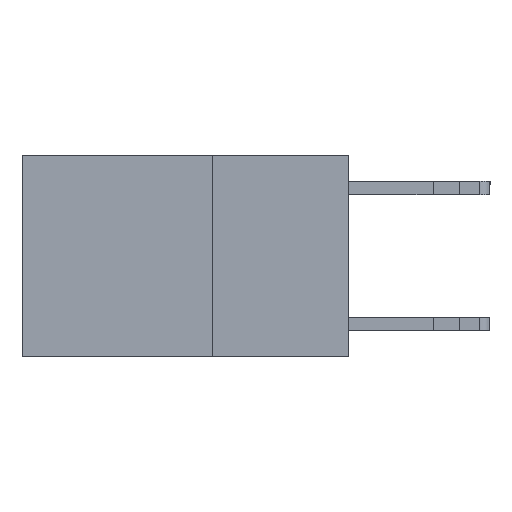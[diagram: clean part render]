
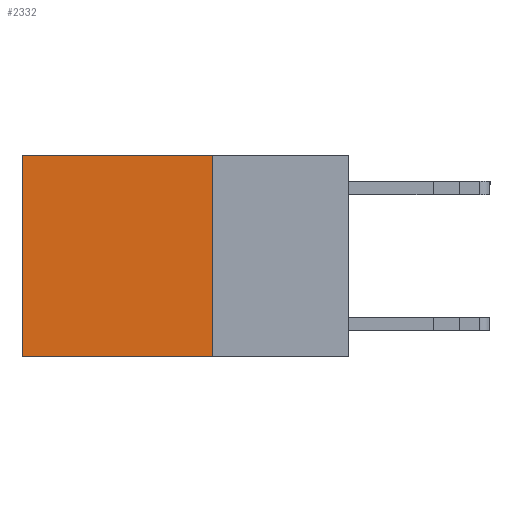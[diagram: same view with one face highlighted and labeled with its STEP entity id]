
A CAD part, left-side view. The second image highlights one B-rep face of the part: STEP entity #2332.
In plain terms, the highlighted planar face has unit normal (-1, 0, 0).
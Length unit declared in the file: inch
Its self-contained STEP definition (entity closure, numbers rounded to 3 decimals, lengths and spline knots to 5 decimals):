
#118 = ORIENTED_EDGE ( 'NONE', *, *, #10918, .F. ) ;
#354 = EDGE_LOOP ( 'NONE', ( #3992, #118, #1312, #5912 ) ) ;
#703 = CARTESIAN_POINT ( 'NONE',  ( 0.2625, 0.25, -0.37 ) ) ;
#1312 = ORIENTED_EDGE ( 'NONE', *, *, #5568, .F. ) ;
#1367 = DIRECTION ( 'NONE',  ( 1., 0., 0. ) ) ;
#1908 = DIRECTION ( 'NONE',  ( 0., 1., 0. ) ) ;
#2332 = ADVANCED_FACE ( 'NONE', ( #8041 ), #6846, .F. ) ;
#2643 = CARTESIAN_POINT ( 'NONE',  ( 0.2625, 0.25, 0. ) ) ;
#2870 = LINE ( 'NONE', #10393, #11684 ) ;
#3019 = EDGE_CURVE ( 'NONE', #7114, #11416, #11569, .T. ) ;
#3902 = AXIS2_PLACEMENT_3D ( 'NONE', #2643, #1367, #10035 ) ;
#3992 = ORIENTED_EDGE ( 'NONE', *, *, #6946, .T. ) ;
#4894 = DIRECTION ( 'NONE',  ( 0., 1., 0. ) ) ;
#5568 = EDGE_CURVE ( 'NONE', #7114, #9580, #7839, .T. ) ;
#5912 = ORIENTED_EDGE ( 'NONE', *, *, #3019, .T. ) ;
#6136 = DIRECTION ( 'NONE',  ( 0., 0., -1. ) ) ;
#6617 = VECTOR ( 'NONE', #11100, 39.37008 ) ;
#6784 = CARTESIAN_POINT ( 'NONE',  ( 0.2625, 0.25, 0. ) ) ;
#6846 = PLANE ( 'NONE',  #3902 ) ;
#6946 = EDGE_CURVE ( 'NONE', #11416, #12065, #2870, .T. ) ;
#7114 = VERTEX_POINT ( 'NONE', #9755 ) ;
#7839 = LINE ( 'NONE', #6784, #6617 ) ;
#8041 = FACE_OUTER_BOUND ( 'NONE', #354, .T. ) ;
#8136 = CARTESIAN_POINT ( 'NONE',  ( 0.2625, 0.6, -0.37 ) ) ;
#9580 = VERTEX_POINT ( 'NONE', #13785 ) ;
#9755 = CARTESIAN_POINT ( 'NONE',  ( 0.2625, 0.25, 0. ) ) ;
#9926 = VECTOR ( 'NONE', #4894, 39.37008 ) ;
#10035 = DIRECTION ( 'NONE',  ( 0., 0., -1. ) ) ;
#10393 = CARTESIAN_POINT ( 'NONE',  ( 0.2625, 0.6, 0. ) ) ;
#10417 = CARTESIAN_POINT ( 'NONE',  ( 0.2625, 0.6, 0. ) ) ;
#10800 = VECTOR ( 'NONE', #1908, 39.37008 ) ;
#10918 = EDGE_CURVE ( 'NONE', #9580, #12065, #12635, .T. ) ;
#11100 = DIRECTION ( 'NONE',  ( 0., 0., -1. ) ) ;
#11416 = VERTEX_POINT ( 'NONE', #10417 ) ;
#11569 = LINE ( 'NONE', #13723, #9926 ) ;
#11684 = VECTOR ( 'NONE', #6136, 39.37008 ) ;
#12065 = VERTEX_POINT ( 'NONE', #8136 ) ;
#12635 = LINE ( 'NONE', #703, #10800 ) ;
#13723 = CARTESIAN_POINT ( 'NONE',  ( 0.2625, 0.25, 0. ) ) ;
#13785 = CARTESIAN_POINT ( 'NONE',  ( 0.2625, 0.25, -0.37 ) ) ;
